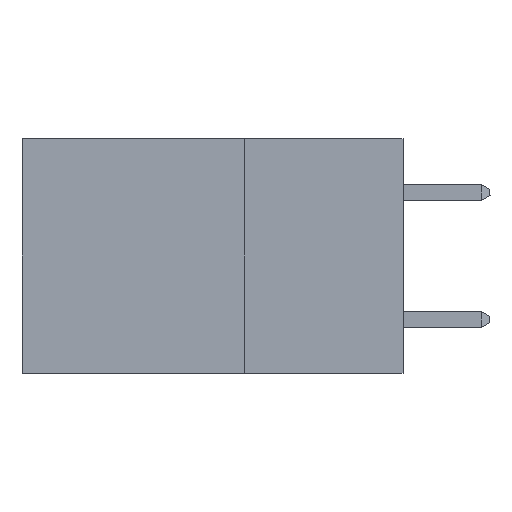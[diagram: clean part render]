
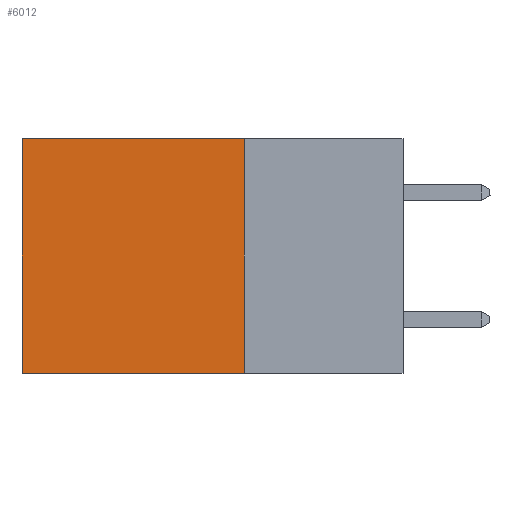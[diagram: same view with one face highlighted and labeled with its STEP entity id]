
A CAD part, left-side view. The second image highlights one B-rep face of the part: STEP entity #6012.
In plain terms, the highlighted planar face has unit normal (-1, 0, 0).
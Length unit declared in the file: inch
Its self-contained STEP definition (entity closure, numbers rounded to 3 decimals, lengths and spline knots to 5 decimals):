
#446 = DIRECTION ( 'NONE',  ( 0., 0., -1. ) ) ;
#802 = ORIENTED_EDGE ( 'NONE', *, *, #10726, .T. ) ;
#1436 = VERTEX_POINT ( 'NONE', #4248 ) ;
#1979 = ORIENTED_EDGE ( 'NONE', *, *, #4342, .F. ) ;
#2250 = DIRECTION ( 'NONE',  ( 0., 1., 0. ) ) ;
#3192 = FACE_OUTER_BOUND ( 'NONE', #14967, .T. ) ;
#3957 = CARTESIAN_POINT ( 'NONE',  ( 0.2875, 0.25, 0. ) ) ;
#4248 = CARTESIAN_POINT ( 'NONE',  ( 0.2875, 0.25, 0. ) ) ;
#4342 = EDGE_CURVE ( 'NONE', #1436, #5836, #6332, .T. ) ;
#4638 = VECTOR ( 'NONE', #446, 39.37008 ) ;
#4924 = VERTEX_POINT ( 'NONE', #5384 ) ;
#5102 = EDGE_CURVE ( 'NONE', #5836, #9719, #10842, .T. ) ;
#5384 = CARTESIAN_POINT ( 'NONE',  ( 0.2875, 0.6, 0. ) ) ;
#5715 = PLANE ( 'NONE',  #11883 ) ;
#5836 = VERTEX_POINT ( 'NONE', #10738 ) ;
#6012 = ADVANCED_FACE ( 'NONE', ( #3192 ), #5715, .F. ) ;
#6332 = LINE ( 'NONE', #3957, #6343 ) ;
#6343 = VECTOR ( 'NONE', #8655, 39.37008 ) ;
#6370 = VECTOR ( 'NONE', #13062, 39.37008 ) ;
#8129 = DIRECTION ( 'NONE',  ( 0., 0., -1. ) ) ;
#8201 = VECTOR ( 'NONE', #2250, 39.37008 ) ;
#8484 = EDGE_CURVE ( 'NONE', #4924, #9719, #12072, .T. ) ;
#8655 = DIRECTION ( 'NONE',  ( 0., 0., -1. ) ) ;
#9271 = DIRECTION ( 'NONE',  ( 1., 0., 0. ) ) ;
#9719 = VERTEX_POINT ( 'NONE', #12450 ) ;
#10726 = EDGE_CURVE ( 'NONE', #1436, #4924, #14177, .T. ) ;
#10738 = CARTESIAN_POINT ( 'NONE',  ( 0.2875, 0.25, -0.37 ) ) ;
#10842 = LINE ( 'NONE', #13368, #6370 ) ;
#11140 = CARTESIAN_POINT ( 'NONE',  ( 0.2875, 0.6, 0. ) ) ;
#11718 = ORIENTED_EDGE ( 'NONE', *, *, #8484, .T. ) ;
#11883 = AXIS2_PLACEMENT_3D ( 'NONE', #12563, #9271, #8129 ) ;
#12072 = LINE ( 'NONE', #11140, #4638 ) ;
#12450 = CARTESIAN_POINT ( 'NONE',  ( 0.2875, 0.6, -0.37 ) ) ;
#12563 = CARTESIAN_POINT ( 'NONE',  ( 0.2875, 0.25, 0. ) ) ;
#13062 = DIRECTION ( 'NONE',  ( 0., 1., 0. ) ) ;
#13368 = CARTESIAN_POINT ( 'NONE',  ( 0.2875, 0.25, -0.37 ) ) ;
#14024 = CARTESIAN_POINT ( 'NONE',  ( 0.2875, 0.25, 0. ) ) ;
#14177 = LINE ( 'NONE', #14024, #8201 ) ;
#14253 = ORIENTED_EDGE ( 'NONE', *, *, #5102, .F. ) ;
#14967 = EDGE_LOOP ( 'NONE', ( #11718, #14253, #1979, #802 ) ) ;
